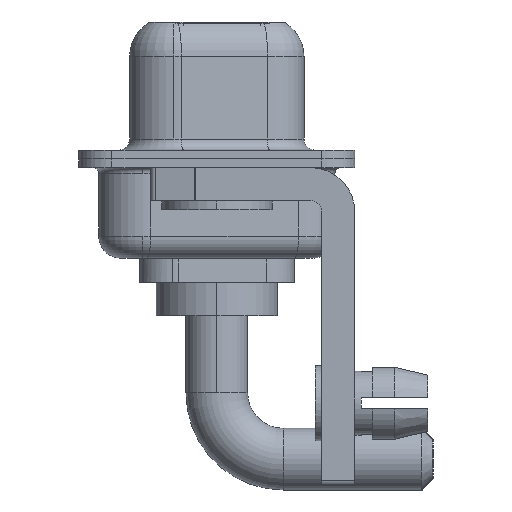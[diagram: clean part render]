
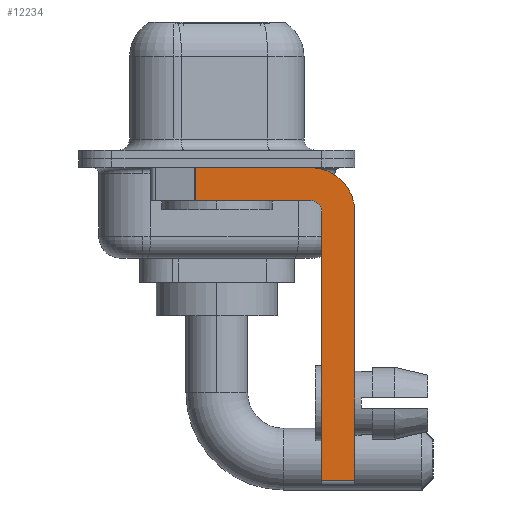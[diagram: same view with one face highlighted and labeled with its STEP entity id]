
A CAD part, left-side view. The second image highlights one B-rep face of the part: STEP entity #12234.
In plain terms, the highlighted planar face has unit normal (-1, 0, 0).
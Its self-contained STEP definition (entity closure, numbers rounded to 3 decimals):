
#315 = CARTESIAN_POINT ( 'NONE',  ( -2.9, 3., -0.4 ) ) ;
#455 = LINE ( 'NONE', #4126, #9651 ) ;
#573 = LINE ( 'NONE', #10420, #14688 ) ;
#739 = EDGE_CURVE ( 'NONE', #7337, #11167, #13860, .T. ) ;
#1232 = LINE ( 'NONE', #13307, #12966 ) ;
#1829 = DIRECTION ( 'NONE',  ( 0., 0., -1. ) ) ;
#2426 = ORIENTED_EDGE ( 'NONE', *, *, #10140, .T. ) ;
#2799 = EDGE_CURVE ( 'NONE', #7974, #10630, #11696, .T. ) ;
#3105 = EDGE_CURVE ( 'NONE', #10630, #4102, #9340, .T. ) ;
#3633 = DIRECTION ( 'NONE',  ( 1., 0., 0. ) ) ;
#4102 = VERTEX_POINT ( 'NONE', #13734 ) ;
#4120 = CARTESIAN_POINT ( 'NONE',  ( -2.9, -4.25, -1.9 ) ) ;
#4126 = CARTESIAN_POINT ( 'NONE',  ( -2.9, 0.978, -1.9 ) ) ;
#4269 = CARTESIAN_POINT ( 'NONE',  ( -2.9, -4.25, -2.4 ) ) ;
#4578 = ORIENTED_EDGE ( 'NONE', *, *, #739, .F. ) ;
#4707 = CARTESIAN_POINT ( 'NONE',  ( -2.9, -4.75, -14.55 ) ) ;
#4905 = EDGE_CURVE ( 'NONE', #7974, #15545, #1232, .T. ) ;
#6075 = CARTESIAN_POINT ( 'NONE',  ( -2.9, -4.25, -2.4 ) ) ;
#6372 = CARTESIAN_POINT ( 'NONE',  ( -2.9, -6.25, -2.4 ) ) ;
#6644 = FACE_OUTER_BOUND ( 'NONE', #8604, .T. ) ;
#7032 = CARTESIAN_POINT ( 'NONE',  ( -2.9, -6.25, -14.55 ) ) ;
#7337 = VERTEX_POINT ( 'NONE', #13918 ) ;
#7493 = DIRECTION ( 'NONE',  ( 0., -1., 0. ) ) ;
#7618 = DIRECTION ( 'NONE',  ( 0., -1., 0. ) ) ;
#7679 = DIRECTION ( 'NONE',  ( 0., 1., 0. ) ) ;
#7707 = VECTOR ( 'NONE', #7679, 1000. ) ;
#7734 = EDGE_CURVE ( 'NONE', #11167, #15545, #573, .T. ) ;
#7974 = VERTEX_POINT ( 'NONE', #4707 ) ;
#8538 = CARTESIAN_POINT ( 'NONE',  ( -2.9, -4.25, -2.4 ) ) ;
#8604 = EDGE_LOOP ( 'NONE', ( #13699, #2426, #8763, #11211, #10652, #8687, #13547, #4578 ) ) ;
#8687 = ORIENTED_EDGE ( 'NONE', *, *, #4905, .T. ) ;
#8763 = ORIENTED_EDGE ( 'NONE', *, *, #14852, .F. ) ;
#9340 = CIRCLE ( 'NONE', #11143, 0.5 ) ;
#9651 = VECTOR ( 'NONE', #1829, 1000. ) ;
#9933 = AXIS2_PLACEMENT_3D ( 'NONE', #4269, #13568, #11193 ) ;
#10073 = CARTESIAN_POINT ( 'NONE',  ( -2.9, 0.978, -1.9 ) ) ;
#10140 = EDGE_CURVE ( 'NONE', #11124, #14891, #455, .T. ) ;
#10420 = CARTESIAN_POINT ( 'NONE',  ( -2.9, -6.25, -2.4 ) ) ;
#10630 = VERTEX_POINT ( 'NONE', #13092 ) ;
#10652 = ORIENTED_EDGE ( 'NONE', *, *, #2799, .F. ) ;
#11124 = VERTEX_POINT ( 'NONE', #12185 ) ;
#11143 = AXIS2_PLACEMENT_3D ( 'NONE', #8538, #12137, #14418 ) ;
#11167 = VERTEX_POINT ( 'NONE', #6372 ) ;
#11193 = DIRECTION ( 'NONE',  ( 0., 0., -1. ) ) ;
#11211 = ORIENTED_EDGE ( 'NONE', *, *, #3105, .F. ) ;
#11696 = LINE ( 'NONE', #14144, #14896 ) ;
#12137 = DIRECTION ( 'NONE',  ( -1., 0., 0. ) ) ;
#12185 = CARTESIAN_POINT ( 'NONE',  ( -2.9, 0.978, -0.4 ) ) ;
#12234 = ADVANCED_FACE ( 'NONE', ( #6644 ), #15132, .F. ) ;
#12313 = LINE ( 'NONE', #4120, #7707 ) ;
#12966 = VECTOR ( 'NONE', #7493, 1000. ) ;
#13031 = DIRECTION ( 'NONE',  ( 0., 0., 1. ) ) ;
#13034 = VECTOR ( 'NONE', #7618, 1000. ) ;
#13092 = CARTESIAN_POINT ( 'NONE',  ( -2.9, -4.75, -2.4 ) ) ;
#13095 = AXIS2_PLACEMENT_3D ( 'NONE', #6075, #3633, #14735 ) ;
#13307 = CARTESIAN_POINT ( 'NONE',  ( -2.9, -4.25, -14.55 ) ) ;
#13547 = ORIENTED_EDGE ( 'NONE', *, *, #7734, .F. ) ;
#13568 = DIRECTION ( 'NONE',  ( 1., 0., 0. ) ) ;
#13596 = LINE ( 'NONE', #315, #13034 ) ;
#13699 = ORIENTED_EDGE ( 'NONE', *, *, #14420, .F. ) ;
#13734 = CARTESIAN_POINT ( 'NONE',  ( -2.9, -4.25, -1.9 ) ) ;
#13860 = CIRCLE ( 'NONE', #13095, 2. ) ;
#13918 = CARTESIAN_POINT ( 'NONE',  ( -2.9, -4.25, -0.4 ) ) ;
#14144 = CARTESIAN_POINT ( 'NONE',  ( -2.9, -4.75, -14.8 ) ) ;
#14418 = DIRECTION ( 'NONE',  ( 0., 0., 1. ) ) ;
#14420 = EDGE_CURVE ( 'NONE', #11124, #7337, #13596, .T. ) ;
#14688 = VECTOR ( 'NONE', #15099, 1000. ) ;
#14735 = DIRECTION ( 'NONE',  ( 0., 0., -1. ) ) ;
#14852 = EDGE_CURVE ( 'NONE', #4102, #14891, #12313, .T. ) ;
#14891 = VERTEX_POINT ( 'NONE', #10073 ) ;
#14896 = VECTOR ( 'NONE', #13031, 1000. ) ;
#15099 = DIRECTION ( 'NONE',  ( 0., 0., -1. ) ) ;
#15132 = PLANE ( 'NONE',  #9933 ) ;
#15545 = VERTEX_POINT ( 'NONE', #7032 ) ;
